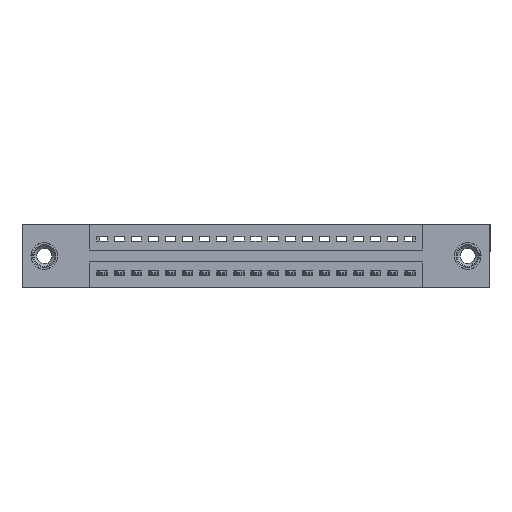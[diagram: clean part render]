
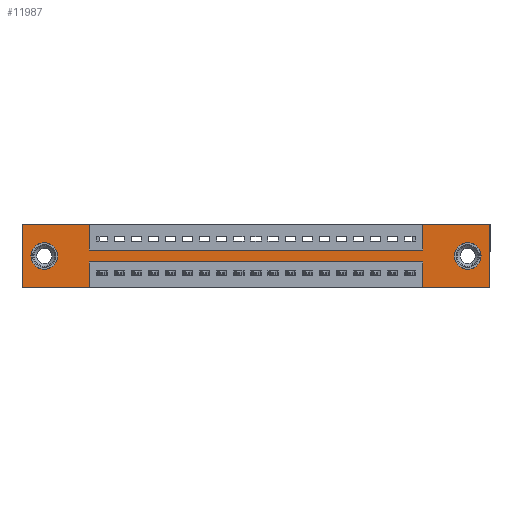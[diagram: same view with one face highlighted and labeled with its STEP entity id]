
A CAD part, front view. The second image highlights one B-rep face of the part: STEP entity #11987.
In plain terms, the highlighted planar face has unit normal (0, -1, 0).
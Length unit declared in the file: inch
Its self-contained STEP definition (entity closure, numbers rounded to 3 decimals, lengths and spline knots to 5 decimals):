
#105 = CARTESIAN_POINT ( 'NONE',  ( 2.605, 0., -0.107 ) ) ;
#241 = VERTEX_POINT ( 'NONE', #16209 ) ;
#308 = CARTESIAN_POINT ( 'NONE',  ( 2.3425, 0., 0. ) ) ;
#341 = DIRECTION ( 'NONE',  ( 0., 0., -1. ) ) ;
#476 = LINE ( 'NONE', #2990, #12012 ) ;
#547 = DIRECTION ( 'NONE',  ( 0., 1., 0. ) ) ;
#887 = ORIENTED_EDGE ( 'NONE', *, *, #11752, .F. ) ;
#1066 = ORIENTED_EDGE ( 'NONE', *, *, #15066, .F. ) ;
#1329 = ORIENTED_EDGE ( 'NONE', *, *, #14218, .T. ) ;
#1353 = LINE ( 'NONE', #3032, #19321 ) ;
#1885 = EDGE_CURVE ( 'NONE', #3171, #14720, #4499, .T. ) ;
#2008 = EDGE_LOOP ( 'NONE', ( #1329, #13947 ) ) ;
#2479 = CARTESIAN_POINT ( 'NONE',  ( 0., 0., 0. ) ) ;
#2540 = EDGE_CURVE ( 'NONE', #19168, #3171, #5438, .T. ) ;
#2671 = ORIENTED_EDGE ( 'NONE', *, *, #3990, .T. ) ;
#2826 = CARTESIAN_POINT ( 'NONE',  ( 0.3925, 0., -0.22 ) ) ;
#2990 = CARTESIAN_POINT ( 'NONE',  ( 0., 0., -0.37 ) ) ;
#3032 = CARTESIAN_POINT ( 'NONE',  ( 0.3925, 0., -0.22 ) ) ;
#3171 = VERTEX_POINT ( 'NONE', #18953 ) ;
#3400 = CARTESIAN_POINT ( 'NONE',  ( 2.735, 0., -0.37 ) ) ;
#3519 = CARTESIAN_POINT ( 'NONE',  ( 0.13, 0., -0.185 ) ) ;
#3947 = VERTEX_POINT ( 'NONE', #13972 ) ;
#3990 = EDGE_CURVE ( 'NONE', #3947, #16958, #13187, .T. ) ;
#4499 = LINE ( 'NONE', #19369, #6402 ) ;
#4783 = CIRCLE ( 'NONE', #5735, 0.078 ) ;
#4872 = ORIENTED_EDGE ( 'NONE', *, *, #8947, .F. ) ;
#5086 = CARTESIAN_POINT ( 'NONE',  ( 0., 0., 0. ) ) ;
#5329 = PLANE ( 'NONE',  #15519 ) ;
#5438 = LINE ( 'NONE', #11702, #9698 ) ;
#5544 = DIRECTION ( 'NONE',  ( 0., 0., 1. ) ) ;
#5612 = DIRECTION ( 'NONE',  ( 0., 0., -1. ) ) ;
#5634 = VERTEX_POINT ( 'NONE', #10387 ) ;
#5635 = DIRECTION ( 'NONE',  ( 1., 0., 0. ) ) ;
#5704 = CARTESIAN_POINT ( 'NONE',  ( 0.3925, 0., -0.37 ) ) ;
#5735 = AXIS2_PLACEMENT_3D ( 'NONE', #3519, #17349, #14114 ) ;
#6035 = VECTOR ( 'NONE', #16403, 39.37008 ) ;
#6091 = VERTEX_POINT ( 'NONE', #16137 ) ;
#6218 = DIRECTION ( 'NONE',  ( -1., 0., 0. ) ) ;
#6349 = VECTOR ( 'NONE', #10536, 39.37008 ) ;
#6402 = VECTOR ( 'NONE', #5544, 39.37008 ) ;
#6466 = ORIENTED_EDGE ( 'NONE', *, *, #1885, .F. ) ;
#6892 = VERTEX_POINT ( 'NONE', #7457 ) ;
#7064 = CARTESIAN_POINT ( 'NONE',  ( 2.605, 0., -0.185 ) ) ;
#7295 = VECTOR ( 'NONE', #18536, 39.37008 ) ;
#7380 = DIRECTION ( 'NONE',  ( 0., -1., 0. ) ) ;
#7457 = CARTESIAN_POINT ( 'NONE',  ( 0., 0., -0.37 ) ) ;
#7579 = CARTESIAN_POINT ( 'NONE',  ( 0.3925, 0., 0. ) ) ;
#7715 = FACE_OUTER_BOUND ( 'NONE', #12146, .T. ) ;
#7740 = CARTESIAN_POINT ( 'NONE',  ( 2.3425, 0., -0.37 ) ) ;
#7752 = CARTESIAN_POINT ( 'NONE',  ( 0.3925, 0., -0.15 ) ) ;
#7957 = LINE ( 'NONE', #5086, #10753 ) ;
#8283 = CIRCLE ( 'NONE', #8863, 0.078 ) ;
#8507 = EDGE_CURVE ( 'NONE', #17476, #19168, #11064, .T. ) ;
#8760 = VERTEX_POINT ( 'NONE', #2826 ) ;
#8863 = AXIS2_PLACEMENT_3D ( 'NONE', #12447, #547, #15339 ) ;
#8947 = EDGE_CURVE ( 'NONE', #11172, #12945, #18672, .T. ) ;
#9051 = ORIENTED_EDGE ( 'NONE', *, *, #2540, .F. ) ;
#9089 = EDGE_CURVE ( 'NONE', #12103, #6892, #476, .T. ) ;
#9200 = LINE ( 'NONE', #2479, #6349 ) ;
#9497 = EDGE_CURVE ( 'NONE', #8760, #12103, #13487, .T. ) ;
#9698 = VECTOR ( 'NONE', #5635, 39.37008 ) ;
#9727 = EDGE_CURVE ( 'NONE', #16958, #3947, #8283, .T. ) ;
#9888 = CARTESIAN_POINT ( 'NONE',  ( 0., 0., -0.37 ) ) ;
#10286 = ORIENTED_EDGE ( 'NONE', *, *, #9497, .F. ) ;
#10375 = VECTOR ( 'NONE', #17592, 39.37008 ) ;
#10387 = CARTESIAN_POINT ( 'NONE',  ( 0., 0., 0. ) ) ;
#10536 = DIRECTION ( 'NONE',  ( 0., 0., 1. ) ) ;
#10662 = ORIENTED_EDGE ( 'NONE', *, *, #9727, .T. ) ;
#10753 = VECTOR ( 'NONE', #15721, 39.37008 ) ;
#11006 = LINE ( 'NONE', #16201, #6035 ) ;
#11064 = LINE ( 'NONE', #16956, #7295 ) ;
#11172 = VERTEX_POINT ( 'NONE', #17183 ) ;
#11252 = FACE_BOUND ( 'NONE', #2008, .T. ) ;
#11609 = DIRECTION ( 'NONE',  ( 0., 1., 0. ) ) ;
#11637 = EDGE_CURVE ( 'NONE', #5634, #17476, #7957, .T. ) ;
#11702 = CARTESIAN_POINT ( 'NONE',  ( 0.3925, 0., -0.15 ) ) ;
#11752 = EDGE_CURVE ( 'NONE', #14720, #11172, #11006, .T. ) ;
#11987 = ADVANCED_FACE ( 'NONE', ( #12898, #11252, #7715 ), #5329, .T. ) ;
#12012 = VECTOR ( 'NONE', #15241, 39.37008 ) ;
#12026 = EDGE_CURVE ( 'NONE', #18637, #8760, #1353, .T. ) ;
#12103 = VERTEX_POINT ( 'NONE', #16521 ) ;
#12146 = EDGE_LOOP ( 'NONE', ( #10286, #13054, #1066, #19244, #4872, #887, #6466, #9051, #18975, #17134, #12865, #15161 ) ) ;
#12309 = EDGE_CURVE ( 'NONE', #12945, #6091, #14588, .T. ) ;
#12389 = VERTEX_POINT ( 'NONE', #15738 ) ;
#12447 = CARTESIAN_POINT ( 'NONE',  ( 2.605, 0., -0.185 ) ) ;
#12865 = ORIENTED_EDGE ( 'NONE', *, *, #16608, .F. ) ;
#12898 = FACE_BOUND ( 'NONE', #15767, .T. ) ;
#12945 = VERTEX_POINT ( 'NONE', #3400 ) ;
#13038 = VECTOR ( 'NONE', #18347, 39.37008 ) ;
#13054 = ORIENTED_EDGE ( 'NONE', *, *, #12026, .F. ) ;
#13187 = CIRCLE ( 'NONE', #16166, 0.078 ) ;
#13487 = LINE ( 'NONE', #5704, #14446 ) ;
#13947 = ORIENTED_EDGE ( 'NONE', *, *, #13977, .T. ) ;
#13972 = CARTESIAN_POINT ( 'NONE',  ( 2.605, 0., -0.263 ) ) ;
#13977 = EDGE_CURVE ( 'NONE', #12389, #241, #4783, .T. ) ;
#13995 = LINE ( 'NONE', #7740, #13038 ) ;
#14114 = DIRECTION ( 'NONE',  ( 0., 0., 1. ) ) ;
#14218 = EDGE_CURVE ( 'NONE', #241, #12389, #19231, .T. ) ;
#14446 = VECTOR ( 'NONE', #14703, 39.37008 ) ;
#14588 = LINE ( 'NONE', #18297, #18149 ) ;
#14703 = DIRECTION ( 'NONE',  ( 0., 0., -1. ) ) ;
#14720 = VERTEX_POINT ( 'NONE', #308 ) ;
#14893 = CARTESIAN_POINT ( 'NONE',  ( 2.3425, 0., -0.22 ) ) ;
#15066 = EDGE_CURVE ( 'NONE', #6091, #18637, #13995, .T. ) ;
#15161 = ORIENTED_EDGE ( 'NONE', *, *, #9089, .F. ) ;
#15241 = DIRECTION ( 'NONE',  ( -1., 0., 0. ) ) ;
#15339 = DIRECTION ( 'NONE',  ( 0., 0., -1. ) ) ;
#15382 = DIRECTION ( 'NONE',  ( 0., 0., 1. ) ) ;
#15455 = CARTESIAN_POINT ( 'NONE',  ( 0.13, 0., -0.185 ) ) ;
#15519 = AXIS2_PLACEMENT_3D ( 'NONE', #9888, #7380, #341 ) ;
#15721 = DIRECTION ( 'NONE',  ( 1., 0., 0. ) ) ;
#15738 = CARTESIAN_POINT ( 'NONE',  ( 0.13, 0., -0.263 ) ) ;
#15767 = EDGE_LOOP ( 'NONE', ( #10662, #2671 ) ) ;
#15920 = AXIS2_PLACEMENT_3D ( 'NONE', #15455, #18359, #15382 ) ;
#15939 = DIRECTION ( 'NONE',  ( -1., 0., 0. ) ) ;
#16014 = CARTESIAN_POINT ( 'NONE',  ( 2.735, 0., 0. ) ) ;
#16137 = CARTESIAN_POINT ( 'NONE',  ( 2.3425, 0., -0.37 ) ) ;
#16166 = AXIS2_PLACEMENT_3D ( 'NONE', #7064, #11609, #5612 ) ;
#16201 = CARTESIAN_POINT ( 'NONE',  ( 0., 0., 0. ) ) ;
#16209 = CARTESIAN_POINT ( 'NONE',  ( 0.13, 0., -0.107 ) ) ;
#16403 = DIRECTION ( 'NONE',  ( 1., 0., 0. ) ) ;
#16521 = CARTESIAN_POINT ( 'NONE',  ( 0.3925, 0., -0.37 ) ) ;
#16608 = EDGE_CURVE ( 'NONE', #6892, #5634, #9200, .T. ) ;
#16956 = CARTESIAN_POINT ( 'NONE',  ( 0.3925, 0., 0. ) ) ;
#16958 = VERTEX_POINT ( 'NONE', #105 ) ;
#17134 = ORIENTED_EDGE ( 'NONE', *, *, #11637, .F. ) ;
#17183 = CARTESIAN_POINT ( 'NONE',  ( 2.735, 0., 0. ) ) ;
#17349 = DIRECTION ( 'NONE',  ( 0., 1., 0. ) ) ;
#17476 = VERTEX_POINT ( 'NONE', #7579 ) ;
#17592 = DIRECTION ( 'NONE',  ( 0., 0., -1. ) ) ;
#18149 = VECTOR ( 'NONE', #6218, 39.37008 ) ;
#18297 = CARTESIAN_POINT ( 'NONE',  ( 0., 0., -0.37 ) ) ;
#18347 = DIRECTION ( 'NONE',  ( 0., 0., 1. ) ) ;
#18359 = DIRECTION ( 'NONE',  ( 0., 1., 0. ) ) ;
#18536 = DIRECTION ( 'NONE',  ( 0., 0., -1. ) ) ;
#18637 = VERTEX_POINT ( 'NONE', #14893 ) ;
#18672 = LINE ( 'NONE', #16014, #10375 ) ;
#18953 = CARTESIAN_POINT ( 'NONE',  ( 2.3425, 0., -0.15 ) ) ;
#18975 = ORIENTED_EDGE ( 'NONE', *, *, #8507, .F. ) ;
#19168 = VERTEX_POINT ( 'NONE', #7752 ) ;
#19231 = CIRCLE ( 'NONE', #15920, 0.078 ) ;
#19244 = ORIENTED_EDGE ( 'NONE', *, *, #12309, .F. ) ;
#19321 = VECTOR ( 'NONE', #15939, 39.37008 ) ;
#19369 = CARTESIAN_POINT ( 'NONE',  ( 2.3425, 0., 0. ) ) ;
